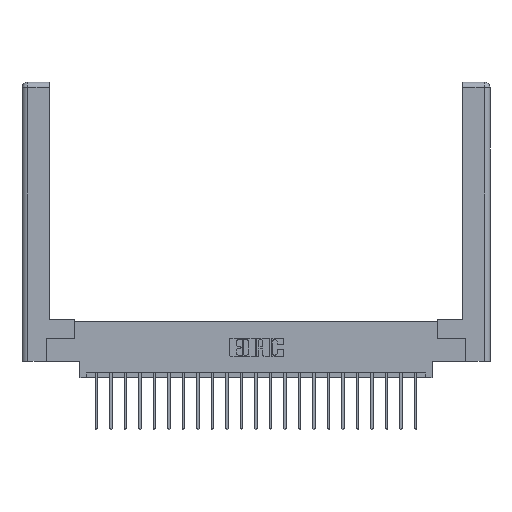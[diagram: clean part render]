
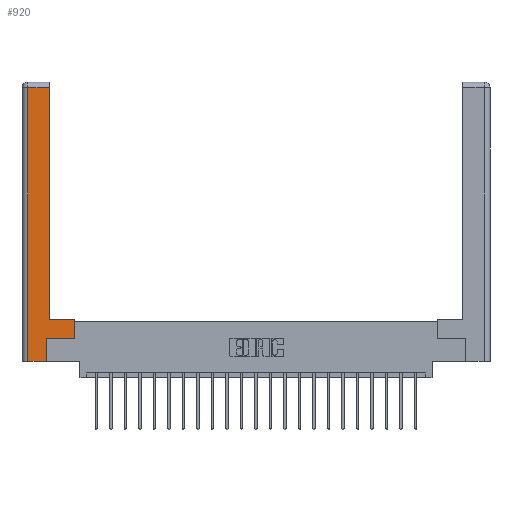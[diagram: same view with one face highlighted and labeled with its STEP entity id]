
A CAD part, top view. The second image highlights one B-rep face of the part: STEP entity #920.
In plain terms, the highlighted planar face has unit normal (0, 0, 1).
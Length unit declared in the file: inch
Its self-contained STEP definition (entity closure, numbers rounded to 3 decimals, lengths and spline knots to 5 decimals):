
#16 = LINE ( 'NONE', #18081, #22910 ) ;
#59 = CARTESIAN_POINT ( 'NONE',  ( 0.265, 0.245, 0. ) ) ;
#570 = ORIENTED_EDGE ( 'NONE', *, *, #909, .T. ) ;
#586 = EDGE_CURVE ( 'NONE', #16751, #8138, #6269, .T. ) ;
#785 = DIRECTION ( 'NONE',  ( 0., 1., 0. ) ) ;
#909 = EDGE_CURVE ( 'NONE', #8138, #1804, #7344, .T. ) ;
#920 = ADVANCED_FACE ( 'NONE', ( #18014 ), #6508, .F. ) ;
#1550 = CARTESIAN_POINT ( 'NONE',  ( 0.0615, 2.94, 0. ) ) ;
#1804 = VERTEX_POINT ( 'NONE', #20517 ) ;
#1813 = CARTESIAN_POINT ( 'NONE',  ( 0.295, 0.45, 0. ) ) ;
#1898 = DIRECTION ( 'NONE',  ( 0., 1., 0. ) ) ;
#1910 = VECTOR ( 'NONE', #1898, 39.37008 ) ;
#2118 = VECTOR ( 'NONE', #7031, 39.37008 ) ;
#2324 = VECTOR ( 'NONE', #7884, 39.37008 ) ;
#2469 = CARTESIAN_POINT ( 'NONE',  ( 0.565, 0.45, 0. ) ) ;
#2522 = VERTEX_POINT ( 'NONE', #15811 ) ;
#3178 = CARTESIAN_POINT ( 'NONE',  ( 0., 0., 0. ) ) ;
#3292 = ORIENTED_EDGE ( 'NONE', *, *, #17001, .T. ) ;
#4707 = CARTESIAN_POINT ( 'NONE',  ( 0.265, 0., 0. ) ) ;
#4947 = DIRECTION ( 'NONE',  ( 0., 0., -1. ) ) ;
#5508 = CARTESIAN_POINT ( 'NONE',  ( 0.0615, 2.94, 0. ) ) ;
#5649 = AXIS2_PLACEMENT_3D ( 'NONE', #3178, #4947, #15779 ) ;
#5722 = CARTESIAN_POINT ( 'NONE',  ( 0.565, 0.245, 0. ) ) ;
#6269 = LINE ( 'NONE', #11353, #2324 ) ;
#6357 = EDGE_LOOP ( 'NONE', ( #17631, #11689, #17320, #570, #20597, #10057, #18845, #3292 ) ) ;
#6508 = PLANE ( 'NONE',  #5649 ) ;
#6928 = CARTESIAN_POINT ( 'NONE',  ( 0.295, 0.45, 0. ) ) ;
#7031 = DIRECTION ( 'NONE',  ( 0., 1., 0. ) ) ;
#7125 = EDGE_CURVE ( 'NONE', #2522, #16751, #17420, .T. ) ;
#7344 = LINE ( 'NONE', #4707, #19926 ) ;
#7884 = DIRECTION ( 'NONE',  ( 0., -1., 0. ) ) ;
#8138 = VERTEX_POINT ( 'NONE', #19370 ) ;
#9449 = EDGE_CURVE ( 'NONE', #1804, #15237, #10348, .T. ) ;
#10057 = ORIENTED_EDGE ( 'NONE', *, *, #16167, .T. ) ;
#10285 = LINE ( 'NONE', #14035, #2118 ) ;
#10323 = LINE ( 'NONE', #5722, #16212 ) ;
#10348 = LINE ( 'NONE', #59, #1910 ) ;
#11353 = CARTESIAN_POINT ( 'NONE',  ( 0.0615, 0., 0. ) ) ;
#11427 = EDGE_CURVE ( 'NONE', #13056, #2522, #10285, .T. ) ;
#11689 = ORIENTED_EDGE ( 'NONE', *, *, #7125, .T. ) ;
#12352 = DIRECTION ( 'NONE',  ( -1., 0., 0. ) ) ;
#13056 = VERTEX_POINT ( 'NONE', #1813 ) ;
#13812 = DIRECTION ( 'NONE',  ( 1., 0., 0. ) ) ;
#14035 = CARTESIAN_POINT ( 'NONE',  ( 0.295, 3., 0. ) ) ;
#14210 = CARTESIAN_POINT ( 'NONE',  ( 0.265, 0.245, 0. ) ) ;
#14535 = DIRECTION ( 'NONE',  ( 1., 0., 0. ) ) ;
#14618 = EDGE_CURVE ( 'NONE', #20762, #22342, #16, .T. ) ;
#15078 = VECTOR ( 'NONE', #12352, 39.37008 ) ;
#15237 = VERTEX_POINT ( 'NONE', #14210 ) ;
#15779 = DIRECTION ( 'NONE',  ( -1., 0., 0. ) ) ;
#15811 = CARTESIAN_POINT ( 'NONE',  ( 0.295, 2.94, 0. ) ) ;
#16167 = EDGE_CURVE ( 'NONE', #15237, #20762, #10323, .T. ) ;
#16212 = VECTOR ( 'NONE', #14535, 39.37008 ) ;
#16751 = VERTEX_POINT ( 'NONE', #1550 ) ;
#17001 = EDGE_CURVE ( 'NONE', #22342, #13056, #19735, .T. ) ;
#17320 = ORIENTED_EDGE ( 'NONE', *, *, #586, .T. ) ;
#17420 = LINE ( 'NONE', #5508, #18807 ) ;
#17631 = ORIENTED_EDGE ( 'NONE', *, *, #11427, .T. ) ;
#18014 = FACE_OUTER_BOUND ( 'NONE', #6357, .T. ) ;
#18081 = CARTESIAN_POINT ( 'NONE',  ( 0.565, 0.45, 0. ) ) ;
#18807 = VECTOR ( 'NONE', #21426, 39.37008 ) ;
#18845 = ORIENTED_EDGE ( 'NONE', *, *, #14618, .T. ) ;
#19328 = CARTESIAN_POINT ( 'NONE',  ( 0.565, 0.245, 0. ) ) ;
#19370 = CARTESIAN_POINT ( 'NONE',  ( 0.0615, 0., 0. ) ) ;
#19735 = LINE ( 'NONE', #6928, #15078 ) ;
#19926 = VECTOR ( 'NONE', #13812, 39.37008 ) ;
#20517 = CARTESIAN_POINT ( 'NONE',  ( 0.265, 0., 0. ) ) ;
#20597 = ORIENTED_EDGE ( 'NONE', *, *, #9449, .T. ) ;
#20762 = VERTEX_POINT ( 'NONE', #19328 ) ;
#21426 = DIRECTION ( 'NONE',  ( -1., 0., 0. ) ) ;
#22342 = VERTEX_POINT ( 'NONE', #2469 ) ;
#22910 = VECTOR ( 'NONE', #785, 39.37008 ) ;
